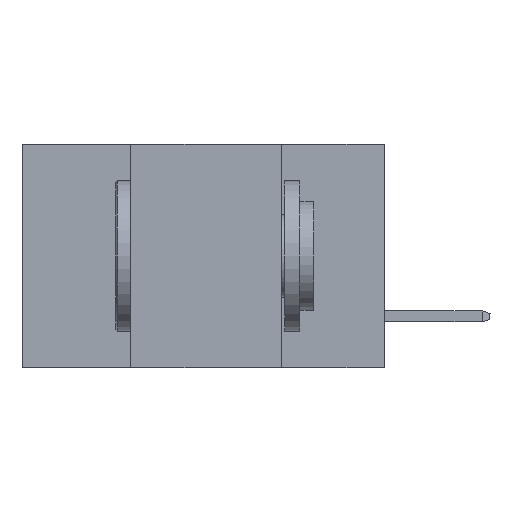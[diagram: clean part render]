
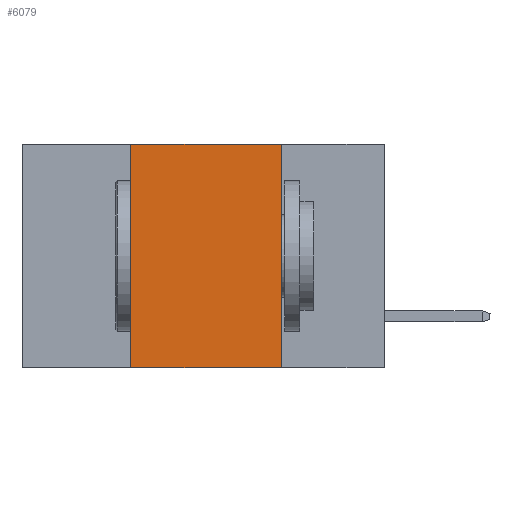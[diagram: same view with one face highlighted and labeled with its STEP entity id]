
A CAD part, left-side view. The second image highlights one B-rep face of the part: STEP entity #6079.
In plain terms, the highlighted planar face has unit normal (-1, 0, 0).
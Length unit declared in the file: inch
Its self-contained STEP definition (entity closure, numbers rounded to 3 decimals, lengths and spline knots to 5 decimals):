
#618 = VECTOR ( 'NONE', #9461, 39.37008 ) ;
#1314 = VERTEX_POINT ( 'NONE', #3046 ) ;
#2123 = PLANE ( 'NONE',  #2613 ) ;
#2196 = CARTESIAN_POINT ( 'NONE',  ( 0., 0.17, -0.37 ) ) ;
#2241 = ORIENTED_EDGE ( 'NONE', *, *, #3562, .T. ) ;
#2419 = DIRECTION ( 'NONE',  ( 0., -1., 0. ) ) ;
#2613 = AXIS2_PLACEMENT_3D ( 'NONE', #8855, #6361, #5495 ) ;
#2962 = FACE_OUTER_BOUND ( 'NONE', #10672, .T. ) ;
#3046 = CARTESIAN_POINT ( 'NONE',  ( 0., 0.42, -0.37 ) ) ;
#3419 = CARTESIAN_POINT ( 'NONE',  ( 0., 0.6, -0.37 ) ) ;
#3562 = EDGE_CURVE ( 'NONE', #1314, #7077, #10246, .T. ) ;
#4414 = DIRECTION ( 'NONE',  ( 0., -1., 0. ) ) ;
#4609 = ORIENTED_EDGE ( 'NONE', *, *, #9749, .F. ) ;
#5045 = ORIENTED_EDGE ( 'NONE', *, *, #8529, .F. ) ;
#5155 = DIRECTION ( 'NONE',  ( 0., 0., -1. ) ) ;
#5334 = VERTEX_POINT ( 'NONE', #8009 ) ;
#5466 = LINE ( 'NONE', #9656, #6875 ) ;
#5495 = DIRECTION ( 'NONE',  ( 0., 0., -1. ) ) ;
#5722 = ORIENTED_EDGE ( 'NONE', *, *, #7294, .F. ) ;
#6079 = ADVANCED_FACE ( 'NONE', ( #2962 ), #2123, .F. ) ;
#6241 = LINE ( 'NONE', #8788, #618 ) ;
#6361 = DIRECTION ( 'NONE',  ( 1., 0., 0. ) ) ;
#6875 = VECTOR ( 'NONE', #4414, 39.37008 ) ;
#7077 = VERTEX_POINT ( 'NONE', #2196 ) ;
#7294 = EDGE_CURVE ( 'NONE', #1314, #9948, #6241, .T. ) ;
#7764 = CARTESIAN_POINT ( 'NONE',  ( 0., 0.17, -0.37 ) ) ;
#8009 = CARTESIAN_POINT ( 'NONE',  ( 0., 0.17, 0. ) ) ;
#8529 = EDGE_CURVE ( 'NONE', #5334, #7077, #10214, .T. ) ;
#8788 = CARTESIAN_POINT ( 'NONE',  ( 0., 0.42, -0.37 ) ) ;
#8855 = CARTESIAN_POINT ( 'NONE',  ( 0., 0.6, 0. ) ) ;
#9196 = VECTOR ( 'NONE', #2419, 39.37008 ) ;
#9220 = CARTESIAN_POINT ( 'NONE',  ( 0., 0.42, 0. ) ) ;
#9412 = VECTOR ( 'NONE', #5155, 39.37008 ) ;
#9461 = DIRECTION ( 'NONE',  ( 0., 0., 1. ) ) ;
#9656 = CARTESIAN_POINT ( 'NONE',  ( 0., 0.6, 0. ) ) ;
#9749 = EDGE_CURVE ( 'NONE', #9948, #5334, #5466, .T. ) ;
#9948 = VERTEX_POINT ( 'NONE', #9220 ) ;
#10214 = LINE ( 'NONE', #7764, #9412 ) ;
#10246 = LINE ( 'NONE', #3419, #9196 ) ;
#10672 = EDGE_LOOP ( 'NONE', ( #5045, #4609, #5722, #2241 ) ) ;
